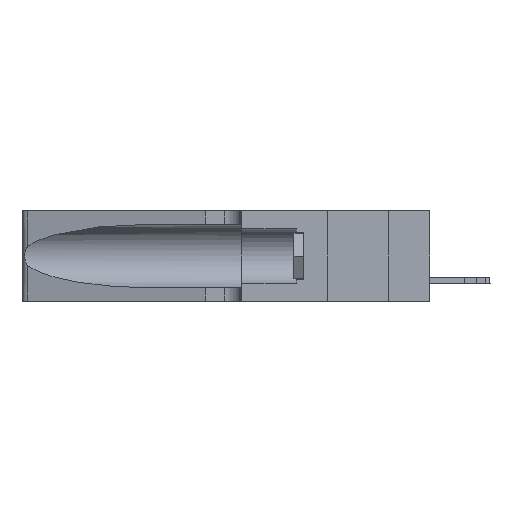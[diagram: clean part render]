
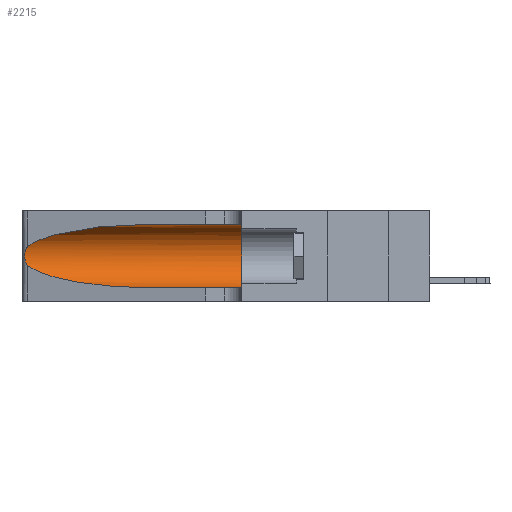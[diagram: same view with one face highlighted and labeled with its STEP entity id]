
A CAD part, left-side view. The second image highlights one B-rep face of the part: STEP entity #2215.
In plain terms, the highlighted cylindrical face has radius 3.308 mm (diameter 6.617 mm), a partial arc.
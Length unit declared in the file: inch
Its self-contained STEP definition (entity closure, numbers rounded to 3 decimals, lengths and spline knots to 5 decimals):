
#115 = LINE ( 'NONE', #706, #9212 ) ;
#616 = AXIS2_PLACEMENT_3D ( 'NONE', #16557, #8418, #5138 ) ;
#661 = ORIENTED_EDGE ( 'NONE', *, *, #1397, .T. ) ;
#706 = CARTESIAN_POINT ( 'NONE',  ( 0.1305, 1.61858, 0.31525 ) ) ;
#1054 = VERTEX_POINT ( 'NONE', #9483 ) ;
#1397 = EDGE_CURVE ( 'NONE', #1054, #8525, #2071, .T. ) ;
#1432 = EDGE_CURVE ( 'NONE', #18609, #15476, #15760, .T. ) ;
#2071 =( BOUNDED_CURVE ( )  B_SPLINE_CURVE ( 3, ( #17096, #18710, #12674, #9449 ),
 .UNSPECIFIED., .F., .T. ) 
 B_SPLINE_CURVE_WITH_KNOTS ( ( 4, 4 ),
 ( 1.5708, 2.84003 ),
 .UNSPECIFIED. ) 
 CURVE ( )  GEOMETRIC_REPRESENTATION_ITEM ( )  RATIONAL_B_SPLINE_CURVE ( ( 1., 0.87, 0.87, 1. ) ) 
 REPRESENTATION_ITEM ( '' )  );
#2215 = ADVANCED_FACE ( 'NONE', ( #9352 ), #9841, .F. ) ;
#2422 = CARTESIAN_POINT ( 'NONE',  ( 0.25555, 1.22994, 0.2215 ) ) ;
#2581 = ORIENTED_EDGE ( 'NONE', *, *, #13203, .T. ) ;
#3129 = VERTEX_POINT ( 'NONE', #11180 ) ;
#4065 = ORIENTED_EDGE ( 'NONE', *, *, #1432, .T. ) ;
#4420 = ORIENTED_EDGE ( 'NONE', *, *, #7167, .T. ) ;
#4558 = CARTESIAN_POINT ( 'NONE',  ( 0.25487, 1.22718, 0.14631 ) ) ;
#5138 = DIRECTION ( 'NONE',  ( 0., 0., 1. ) ) ;
#5598 = B_SPLINE_CURVE_WITH_KNOTS ( 'NONE', 3,
 ( #19998, #2422, #13702, #19849, #18516, #11857, #18873, #12205, #7454, #15523, #17797, #18919, #10786, #10929 ),
 .UNSPECIFIED., .F., .F.,
 ( 4, 2, 2, 2, 2, 2, 4 ),
 ( 0., 0.00027, 0.00053, 0.00107, 0.0016, 0.00187, 0.00214 ),
 .UNSPECIFIED. ) ;
#5659 = CARTESIAN_POINT ( 'NONE',  ( 0.25487, 1.22718, 0.14631 ) ) ;
#6344 = LINE ( 'NONE', #14557, #10092 ) ;
#6886 = ORIENTED_EDGE ( 'NONE', *, *, #7607, .F. ) ;
#7167 = EDGE_CURVE ( 'NONE', #15476, #3129, #6344, .T. ) ;
#7454 = CARTESIAN_POINT ( 'NONE',  ( 0.26017, 1.23833, 0.17102 ) ) ;
#7607 = EDGE_CURVE ( 'NONE', #14344, #3129, #11844, .T. ) ;
#7700 = CARTESIAN_POINT ( 'NONE',  ( 0.18966, 0.96281, 0.05475 ) ) ;
#8418 = DIRECTION ( 'NONE',  ( 0., 1., 0. ) ) ;
#8523 = AXIS2_PLACEMENT_3D ( 'NONE', #16869, #18386, #20005 ) ;
#8525 = VERTEX_POINT ( 'NONE', #14946 ) ;
#9212 = VECTOR ( 'NONE', #11845, 39.37008 ) ;
#9302 = CARTESIAN_POINT ( 'NONE',  ( 0.1305, 0.72297, 0.05475 ) ) ;
#9352 = FACE_OUTER_BOUND ( 'NONE', #20161, .T. ) ;
#9449 = CARTESIAN_POINT ( 'NONE',  ( 0.25487, 1.22718, 0.22369 ) ) ;
#9483 = CARTESIAN_POINT ( 'NONE',  ( 0.1305, 0.72297, 0.31525 ) ) ;
#9841 = CYLINDRICAL_SURFACE ( 'NONE', #8523, 0.13025 ) ;
#10092 = VECTOR ( 'NONE', #16166, 39.37008 ) ;
#10164 = CARTESIAN_POINT ( 'NONE',  ( 0.1305, 0.35, 0.31525 ) ) ;
#10786 = CARTESIAN_POINT ( 'NONE',  ( 0.25555, 1.22993, 0.14849 ) ) ;
#10929 = CARTESIAN_POINT ( 'NONE',  ( 0.25487, 1.22718, 0.14631 ) ) ;
#11180 = CARTESIAN_POINT ( 'NONE',  ( 0.1305, 0.35, 0.05475 ) ) ;
#11844 = CIRCLE ( 'NONE', #616, 0.13025 ) ;
#11845 = DIRECTION ( 'NONE',  ( 0., -1., 0. ) ) ;
#11857 = CARTESIAN_POINT ( 'NONE',  ( 0.26018, 1.23835, 0.19895 ) ) ;
#12205 = CARTESIAN_POINT ( 'NONE',  ( 0.26075, 1.23896, 0.178 ) ) ;
#12674 = CARTESIAN_POINT ( 'NONE',  ( 0.2373, 1.15595, 0.28018 ) ) ;
#13203 = EDGE_CURVE ( 'NONE', #8525, #18609, #5598, .T. ) ;
#13702 = CARTESIAN_POINT ( 'NONE',  ( 0.25639, 1.23184, 0.21858 ) ) ;
#14344 = VERTEX_POINT ( 'NONE', #10164 ) ;
#14557 = CARTESIAN_POINT ( 'NONE',  ( 0.1305, 1.61858, 0.05475 ) ) ;
#14841 = CARTESIAN_POINT ( 'NONE',  ( 0.1305, 0.72297, 0.05475 ) ) ;
#14946 = CARTESIAN_POINT ( 'NONE',  ( 0.25487, 1.22718, 0.22369 ) ) ;
#15476 = VERTEX_POINT ( 'NONE', #14841 ) ;
#15523 = CARTESIAN_POINT ( 'NONE',  ( 0.25856, 1.23593, 0.16098 ) ) ;
#15760 =( BOUNDED_CURVE ( )  B_SPLINE_CURVE ( 3, ( #4558, #17247, #7700, #9302 ),
 .UNSPECIFIED., .F., .F. ) 
 B_SPLINE_CURVE_WITH_KNOTS ( ( 4, 4 ),
 ( 3.44316, 4.71239 ),
 .UNSPECIFIED. ) 
 CURVE ( )  GEOMETRIC_REPRESENTATION_ITEM ( )  RATIONAL_B_SPLINE_CURVE ( ( 1., 0.87, 0.87, 1. ) ) 
 REPRESENTATION_ITEM ( '' )  );
#16166 = DIRECTION ( 'NONE',  ( 0., -1., 0. ) ) ;
#16327 = EDGE_CURVE ( 'NONE', #1054, #14344, #115, .T. ) ;
#16557 = CARTESIAN_POINT ( 'NONE',  ( 0.1305, 0.35, 0.185 ) ) ;
#16869 = CARTESIAN_POINT ( 'NONE',  ( 0.1305, 1.61858, 0.185 ) ) ;
#17096 = CARTESIAN_POINT ( 'NONE',  ( 0.1305, 0.72297, 0.31525 ) ) ;
#17247 = CARTESIAN_POINT ( 'NONE',  ( 0.2373, 1.15595, 0.08982 ) ) ;
#17797 = CARTESIAN_POINT ( 'NONE',  ( 0.25789, 1.23486, 0.15765 ) ) ;
#18386 = DIRECTION ( 'NONE',  ( 0., -1., 0. ) ) ;
#18516 = CARTESIAN_POINT ( 'NONE',  ( 0.25854, 1.2359, 0.20912 ) ) ;
#18609 = VERTEX_POINT ( 'NONE', #5659 ) ;
#18710 = CARTESIAN_POINT ( 'NONE',  ( 0.18966, 0.96281, 0.31525 ) ) ;
#18873 = CARTESIAN_POINT ( 'NONE',  ( 0.26075, 1.23896, 0.19203 ) ) ;
#18919 = CARTESIAN_POINT ( 'NONE',  ( 0.25639, 1.23186, 0.15144 ) ) ;
#19849 = CARTESIAN_POINT ( 'NONE',  ( 0.25787, 1.23484, 0.2124 ) ) ;
#19870 = ORIENTED_EDGE ( 'NONE', *, *, #16327, .F. ) ;
#19998 = CARTESIAN_POINT ( 'NONE',  ( 0.25487, 1.22718, 0.22369 ) ) ;
#20005 = DIRECTION ( 'NONE',  ( 0., 0., -1. ) ) ;
#20161 = EDGE_LOOP ( 'NONE', ( #661, #2581, #4065, #4420, #6886, #19870 ) ) ;
